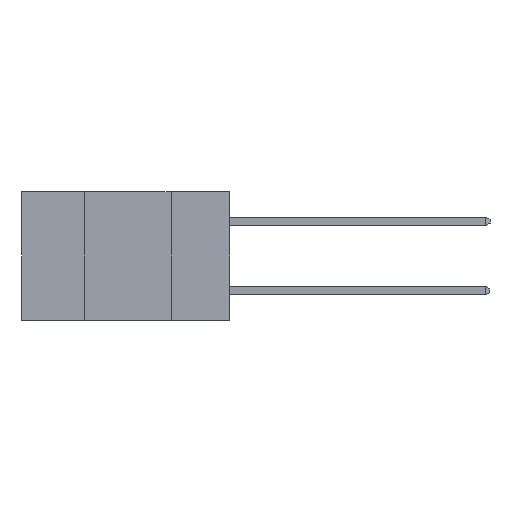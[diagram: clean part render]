
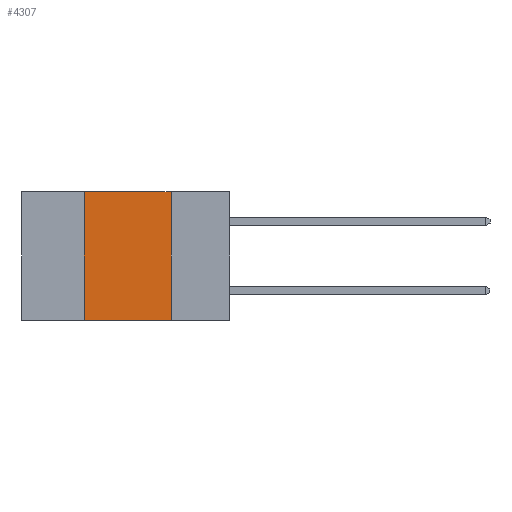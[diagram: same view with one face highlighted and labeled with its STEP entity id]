
A CAD part, left-side view. The second image highlights one B-rep face of the part: STEP entity #4307.
In plain terms, the highlighted planar face has unit normal (-1, 0, 0).
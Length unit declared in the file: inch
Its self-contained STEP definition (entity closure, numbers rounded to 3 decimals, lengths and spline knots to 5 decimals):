
#836 = DIRECTION ( 'NONE',  ( 0., 0., -1. ) ) ;
#1683 = VECTOR ( 'NONE', #24297, 39.37008 ) ;
#1712 = LINE ( 'NONE', #10508, #7542 ) ;
#1822 = VECTOR ( 'NONE', #5006, 39.37008 ) ;
#3453 = EDGE_CURVE ( 'NONE', #19576, #20426, #28096, .T. ) ;
#3778 = AXIS2_PLACEMENT_3D ( 'NONE', #20525, #15667, #836 ) ;
#4307 = ADVANCED_FACE ( 'NONE', ( #14930 ), #10707, .F. ) ;
#5006 = DIRECTION ( 'NONE',  ( 0., -1., 0. ) ) ;
#5072 = LINE ( 'NONE', #23217, #30579 ) ;
#6559 = CARTESIAN_POINT ( 'NONE',  ( 0., 0.42, -0.37 ) ) ;
#7542 = VECTOR ( 'NONE', #30242, 39.37008 ) ;
#8210 = ORIENTED_EDGE ( 'NONE', *, *, #11982, .F. ) ;
#10192 = VERTEX_POINT ( 'NONE', #16652 ) ;
#10508 = CARTESIAN_POINT ( 'NONE',  ( 0., 0.42, 0. ) ) ;
#10707 = PLANE ( 'NONE',  #3778 ) ;
#11982 = EDGE_CURVE ( 'NONE', #19576, #10192, #1712, .T. ) ;
#12404 = EDGE_CURVE ( 'NONE', #12645, #20426, #14858, .T. ) ;
#12645 = VERTEX_POINT ( 'NONE', #22796 ) ;
#13848 = ORIENTED_EDGE ( 'NONE', *, *, #27364, .F. ) ;
#14848 = CARTESIAN_POINT ( 'NONE',  ( 0., 0.17, -0.37 ) ) ;
#14858 = LINE ( 'NONE', #21827, #1683 ) ;
#14930 = FACE_OUTER_BOUND ( 'NONE', #30426, .T. ) ;
#15454 = ORIENTED_EDGE ( 'NONE', *, *, #3453, .T. ) ;
#15667 = DIRECTION ( 'NONE',  ( 1., 0., 0. ) ) ;
#15746 = DIRECTION ( 'NONE',  ( 0., -1., 0. ) ) ;
#16652 = CARTESIAN_POINT ( 'NONE',  ( 0., 0.42, 0. ) ) ;
#17337 = CARTESIAN_POINT ( 'NONE',  ( 0., 0.6, -0.37 ) ) ;
#19576 = VERTEX_POINT ( 'NONE', #6559 ) ;
#20426 = VERTEX_POINT ( 'NONE', #14848 ) ;
#20525 = CARTESIAN_POINT ( 'NONE',  ( 0., 0.6, 0. ) ) ;
#21827 = CARTESIAN_POINT ( 'NONE',  ( 0., 0.17, 0. ) ) ;
#22796 = CARTESIAN_POINT ( 'NONE',  ( 0., 0.17, 0. ) ) ;
#23217 = CARTESIAN_POINT ( 'NONE',  ( 0., 0.6, 0. ) ) ;
#24297 = DIRECTION ( 'NONE',  ( 0., 0., -1. ) ) ;
#27364 = EDGE_CURVE ( 'NONE', #10192, #12645, #5072, .T. ) ;
#28096 = LINE ( 'NONE', #17337, #1822 ) ;
#30242 = DIRECTION ( 'NONE',  ( 0., 0., 1. ) ) ;
#30426 = EDGE_LOOP ( 'NONE', ( #30680, #13848, #8210, #15454 ) ) ;
#30579 = VECTOR ( 'NONE', #15746, 39.37008 ) ;
#30680 = ORIENTED_EDGE ( 'NONE', *, *, #12404, .F. ) ;
